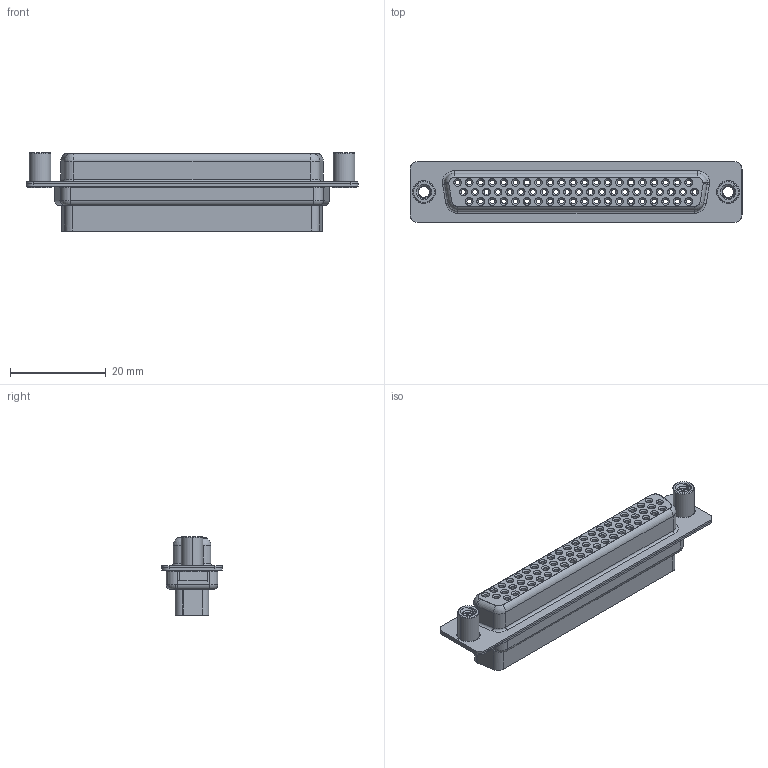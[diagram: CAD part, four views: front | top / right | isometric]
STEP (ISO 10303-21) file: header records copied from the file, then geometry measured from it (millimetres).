
FILE_DESCRIPTION (( 'STEP AP203' ), '1' );
FILE_NAME ('638-062-010-048.STEP', '2020-07-18T16:46:51', ( '' ), ( '' ), 'SwSTEP 2.0', 'SolidWorks 2020', '' );
FILE_SCHEMA (( 'CONFIG_CONTROL_DESIGN' ));
Length unit declared in the file: millimetre
Products named in the file (5): 638 Housing_62 Contacts HP; 638 4-40 Threaded Standoff; 638 Shell Rear_62 Contacts; 638 Shell Front_62 Contacts; 638-062-010-048
Assembly tree (5 placements, depth 2):
  638-062-010-048
    638 Housing_62 Contacts HP
    638 Shell Front_62 Contacts
    638 Shell Rear_62 Contacts
    638 4-40 Threaded Standoff  x2
Bounding box: 69.32 x 12.6 x 16.3 mm (x, y, z)
Volume: 4992.8 mm3; surface area: 13123.5 mm2
Topology: 5 solids, 5 shells, 1119 faces, 2513 edges, 1603 vertices
Faces by surface type: cylinder 661, plane 255, cone 140, torus 57, bspline 6
Entity records: 32621 total; most frequent: CARTESIAN_POINT 6923, DIRECTION 5834, ORIENTED_EDGE 4772, AXIS2_PLACEMENT_3D 2475, EDGE_CURVE 2386, VERTEX_POINT 1521, EDGE_LOOP 1403, CIRCLE 1401
